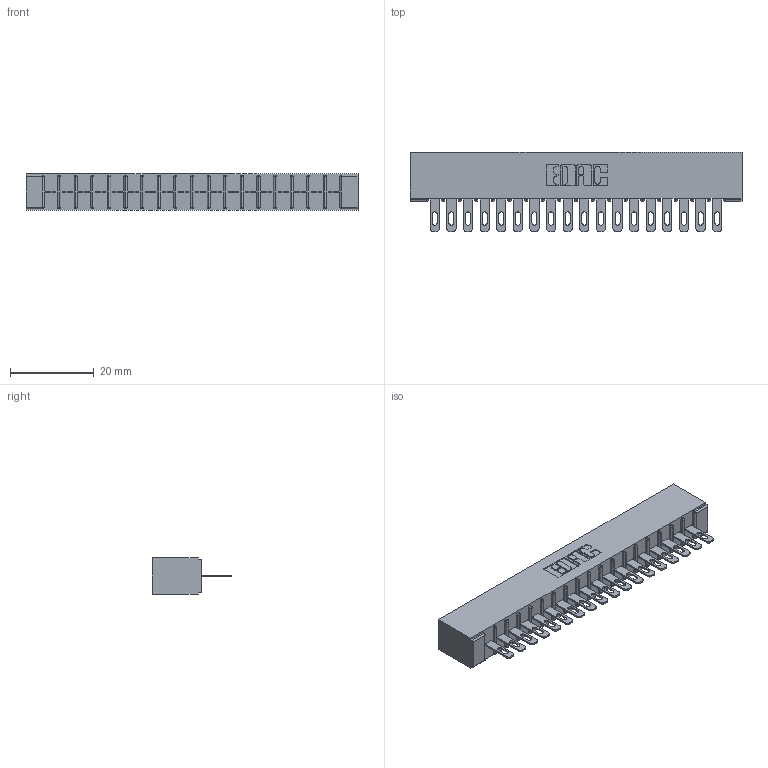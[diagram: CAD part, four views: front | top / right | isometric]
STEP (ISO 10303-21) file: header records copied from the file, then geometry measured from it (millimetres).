
FILE_DESCRIPTION (( 'STEP AP203' ), '1' );
FILE_NAME ('316-018-500-101.STEP', '2018-07-31T01:12:31', ( '' ), ( '' ), 'SwSTEP 2.0', 'SolidWorks 2016', '' );
FILE_SCHEMA (( 'CONFIG_CONTROL_DESIGN' ));
Length unit declared in the file: inch
Products named in the file (3): 316-018-500-101; 306 Part_No Mounting; 306-290-001_100
Assembly tree (19 placements, depth 2):
  316-018-500-101
    306 Part_No Mounting
    306-290-001_100  x18
Bounding box: 79.2 x 18.87 x 8.71 mm (x, y, z)
Volume: 5737.3 mm3; surface area: 8892.3 mm2
Topology: 19 solids, 19 shells, 1476 faces, 4162 edges, 2676 vertices
Faces by surface type: plane 964, cylinder 440, sphere 72
Entity records: 19781 total; most frequent: CARTESIAN_POINT 3317, ORIENTED_EDGE 3284, DIRECTION 3274, EDGE_CURVE 1642, VECTOR 1272, LINE 1272, VERTEX_POINT 1044, AXIS2_PLACEMENT_3D 1001
